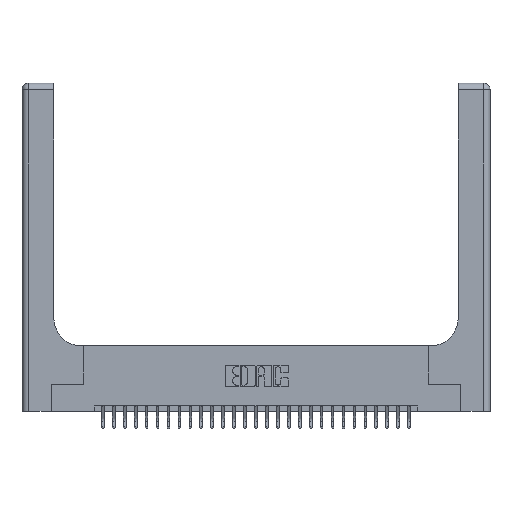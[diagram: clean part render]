
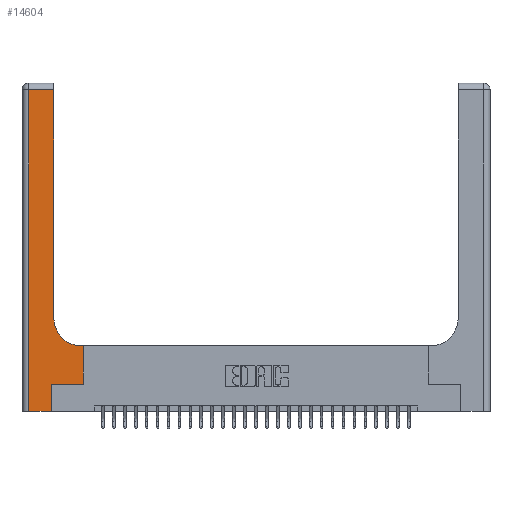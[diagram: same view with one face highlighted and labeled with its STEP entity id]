
A CAD part, top view. The second image highlights one B-rep face of the part: STEP entity #14604.
In plain terms, the highlighted planar face has unit normal (0, 0, 1).
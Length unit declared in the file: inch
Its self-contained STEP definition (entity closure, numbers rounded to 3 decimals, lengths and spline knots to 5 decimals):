
#346 = DIRECTION ( 'NONE',  ( 1., 0., 0. ) ) ;
#391 = CIRCLE ( 'NONE', #2989, 0.25 ) ;
#607 = CARTESIAN_POINT ( 'NONE',  ( 0.2915, 0.6, 0.37 ) ) ;
#807 = CARTESIAN_POINT ( 'NONE',  ( 0., 3., 0.37 ) ) ;
#1374 = ORIENTED_EDGE ( 'NONE', *, *, #9910, .T. ) ;
#1375 = LINE ( 'NONE', #16983, #3152 ) ;
#1737 = CARTESIAN_POINT ( 'NONE',  ( 0.5585, 0.25, 0.37 ) ) ;
#2332 = DIRECTION ( 'NONE',  ( -1., 0., 0. ) ) ;
#2532 = EDGE_CURVE ( 'NONE', #15044, #9689, #6434, .T. ) ;
#2655 = EDGE_CURVE ( 'NONE', #29824, #22834, #13656, .T. ) ;
#2989 = AXIS2_PLACEMENT_3D ( 'NONE', #4220, #6538, #22742 ) ;
#3123 = VERTEX_POINT ( 'NONE', #22548 ) ;
#3152 = VECTOR ( 'NONE', #7778, 39.37008 ) ;
#3981 = CARTESIAN_POINT ( 'NONE',  ( 0., 2.94, 0.37 ) ) ;
#3995 = ORIENTED_EDGE ( 'NONE', *, *, #16259, .T. ) ;
#4220 = CARTESIAN_POINT ( 'NONE',  ( 0.5415, 0.85, 0.37 ) ) ;
#4371 = CARTESIAN_POINT ( 'NONE',  ( 0.06, 2.94, 0.37 ) ) ;
#4505 = CARTESIAN_POINT ( 'NONE',  ( 0.269, 0.25, 0.37 ) ) ;
#4861 = VECTOR ( 'NONE', #2332, 39.37008 ) ;
#6163 = ORIENTED_EDGE ( 'NONE', *, *, #11315, .T. ) ;
#6434 = LINE ( 'NONE', #4505, #11162 ) ;
#6538 = DIRECTION ( 'NONE',  ( 0., 0., -1. ) ) ;
#6554 = EDGE_CURVE ( 'NONE', #28015, #3123, #9794, .T. ) ;
#6926 = LINE ( 'NONE', #25397, #24687 ) ;
#7155 = ORIENTED_EDGE ( 'NONE', *, *, #20675, .T. ) ;
#7443 = ORIENTED_EDGE ( 'NONE', *, *, #2532, .T. ) ;
#7467 = DIRECTION ( 'NONE',  ( 0., 0., -1. ) ) ;
#7778 = DIRECTION ( 'NONE',  ( 0., 1., 0. ) ) ;
#8292 = LINE ( 'NONE', #3981, #29640 ) ;
#9357 = CARTESIAN_POINT ( 'NONE',  ( 0.269, 0.25, 0.37 ) ) ;
#9689 = VERTEX_POINT ( 'NONE', #1737 ) ;
#9784 = DIRECTION ( 'NONE',  ( -1., 0., 0. ) ) ;
#9794 = LINE ( 'NONE', #28303, #22838 ) ;
#9910 = EDGE_CURVE ( 'NONE', #25555, #10357, #12831, .T. ) ;
#10357 = VERTEX_POINT ( 'NONE', #25182 ) ;
#11162 = VECTOR ( 'NONE', #346, 39.37008 ) ;
#11315 = EDGE_CURVE ( 'NONE', #3123, #25010, #21668, .T. ) ;
#12831 = LINE ( 'NONE', #607, #4861 ) ;
#12854 = CARTESIAN_POINT ( 'NONE',  ( 0.2915, 3., 0.37 ) ) ;
#13166 = EDGE_LOOP ( 'NONE', ( #19543, #7155, #14337, #6163, #3995, #7443, #25833, #1374, #16563 ) ) ;
#13656 = LINE ( 'NONE', #12854, #20888 ) ;
#13691 = CARTESIAN_POINT ( 'NONE',  ( 0.5585, 0.6, 0.37 ) ) ;
#14337 = ORIENTED_EDGE ( 'NONE', *, *, #6554, .T. ) ;
#14604 = ADVANCED_FACE ( 'NONE', ( #23627 ), #19164, .F. ) ;
#15044 = VERTEX_POINT ( 'NONE', #9357 ) ;
#15239 = DIRECTION ( 'NONE',  ( 0., -1., 0. ) ) ;
#16259 = EDGE_CURVE ( 'NONE', #25010, #15044, #6926, .T. ) ;
#16563 = ORIENTED_EDGE ( 'NONE', *, *, #19770, .T. ) ;
#16983 = CARTESIAN_POINT ( 'NONE',  ( 0.5585, 0.25, 0.37 ) ) ;
#18113 = CARTESIAN_POINT ( 'NONE',  ( 0., 0., 0.37 ) ) ;
#18685 = DIRECTION ( 'NONE',  ( 0., 1., 0. ) ) ;
#19164 = PLANE ( 'NONE',  #27619 ) ;
#19543 = ORIENTED_EDGE ( 'NONE', *, *, #2655, .T. ) ;
#19770 = EDGE_CURVE ( 'NONE', #10357, #29824, #391, .T. ) ;
#20675 = EDGE_CURVE ( 'NONE', #22834, #28015, #8292, .T. ) ;
#20888 = VECTOR ( 'NONE', #28931, 39.37008 ) ;
#21064 = CARTESIAN_POINT ( 'NONE',  ( 0.2915, 2.94, 0.37 ) ) ;
#21272 = VECTOR ( 'NONE', #29736, 39.37008 ) ;
#21668 = LINE ( 'NONE', #18113, #21272 ) ;
#21850 = EDGE_CURVE ( 'NONE', #9689, #25555, #1375, .T. ) ;
#22548 = CARTESIAN_POINT ( 'NONE',  ( 0.06, 0., 0.37 ) ) ;
#22742 = DIRECTION ( 'NONE',  ( 1., 0., 0. ) ) ;
#22817 = CARTESIAN_POINT ( 'NONE',  ( 0.2915, 0.85, 0.37 ) ) ;
#22834 = VERTEX_POINT ( 'NONE', #21064 ) ;
#22838 = VECTOR ( 'NONE', #15239, 39.37008 ) ;
#23457 = CARTESIAN_POINT ( 'NONE',  ( 0.269, 0., 0.37 ) ) ;
#23627 = FACE_OUTER_BOUND ( 'NONE', #13166, .T. ) ;
#24687 = VECTOR ( 'NONE', #18685, 39.37008 ) ;
#25010 = VERTEX_POINT ( 'NONE', #23457 ) ;
#25182 = CARTESIAN_POINT ( 'NONE',  ( 0.5415, 0.6, 0.37 ) ) ;
#25397 = CARTESIAN_POINT ( 'NONE',  ( 0.269, 0., 0.37 ) ) ;
#25555 = VERTEX_POINT ( 'NONE', #13691 ) ;
#25833 = ORIENTED_EDGE ( 'NONE', *, *, #21850, .T. ) ;
#26755 = DIRECTION ( 'NONE',  ( -1., 0., 0. ) ) ;
#27619 = AXIS2_PLACEMENT_3D ( 'NONE', #807, #7467, #9784 ) ;
#28015 = VERTEX_POINT ( 'NONE', #4371 ) ;
#28303 = CARTESIAN_POINT ( 'NONE',  ( 0.06, 3., 0.37 ) ) ;
#28931 = DIRECTION ( 'NONE',  ( 0., 1., 0. ) ) ;
#29640 = VECTOR ( 'NONE', #26755, 39.37008 ) ;
#29736 = DIRECTION ( 'NONE',  ( 1., 0., 0. ) ) ;
#29824 = VERTEX_POINT ( 'NONE', #22817 ) ;
